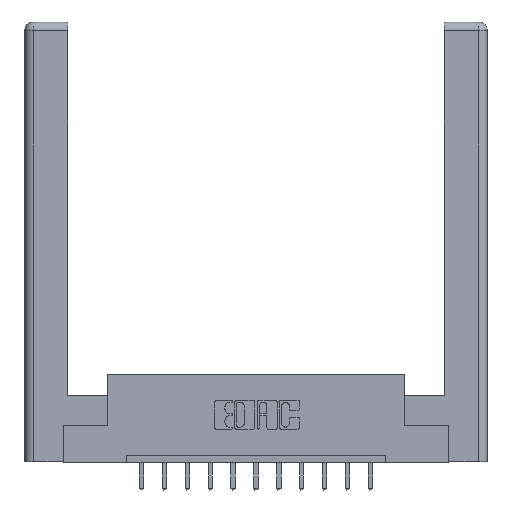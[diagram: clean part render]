
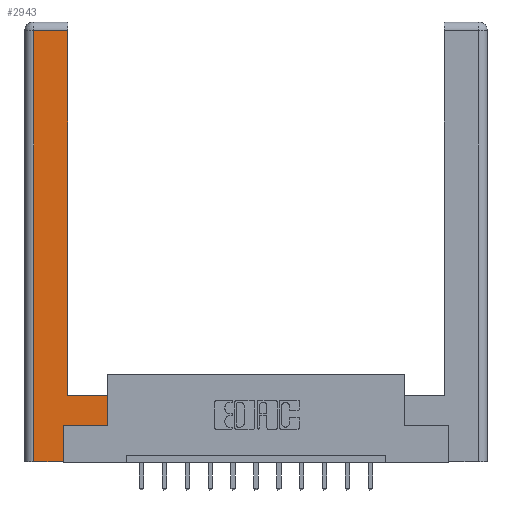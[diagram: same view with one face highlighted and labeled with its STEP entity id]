
A CAD part, top view. The second image highlights one B-rep face of the part: STEP entity #2943.
In plain terms, the highlighted planar face has unit normal (0, 0, 1).
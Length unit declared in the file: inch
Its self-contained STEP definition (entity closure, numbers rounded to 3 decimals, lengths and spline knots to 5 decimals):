
#169 = ORIENTED_EDGE ( 'NONE', *, *, #5644, .T. ) ;
#477 = LINE ( 'NONE', #10671, #6953 ) ;
#510 = CARTESIAN_POINT ( 'NONE',  ( 0.0615, 0., 0. ) ) ;
#787 = ORIENTED_EDGE ( 'NONE', *, *, #1074, .T. ) ;
#793 = DIRECTION ( 'NONE',  ( 0., 1., 0. ) ) ;
#1074 = EDGE_CURVE ( 'NONE', #13514, #2244, #11296, .T. ) ;
#1350 = EDGE_CURVE ( 'NONE', #8315, #7139, #10539, .T. ) ;
#1423 = CARTESIAN_POINT ( 'NONE',  ( 0.565, 0.245, 0. ) ) ;
#1701 = CARTESIAN_POINT ( 'NONE',  ( 0.265, 0.245, 0. ) ) ;
#2244 = VERTEX_POINT ( 'NONE', #6016 ) ;
#2795 = VERTEX_POINT ( 'NONE', #6215 ) ;
#2849 = ORIENTED_EDGE ( 'NONE', *, *, #7097, .T. ) ;
#2943 = ADVANCED_FACE ( 'NONE', ( #5965 ), #5645, .F. ) ;
#3038 = AXIS2_PLACEMENT_3D ( 'NONE', #4341, #6858, #13749 ) ;
#3250 = CARTESIAN_POINT ( 'NONE',  ( 0.265, 0., 0. ) ) ;
#3886 = EDGE_CURVE ( 'NONE', #2244, #4468, #7607, .T. ) ;
#3928 = DIRECTION ( 'NONE',  ( 0., 1., 0. ) ) ;
#4077 = DIRECTION ( 'NONE',  ( 0., -1., 0. ) ) ;
#4226 = LINE ( 'NONE', #6475, #12362 ) ;
#4303 = DIRECTION ( 'NONE',  ( 0., 1., 0. ) ) ;
#4341 = CARTESIAN_POINT ( 'NONE',  ( 0., 0., 0. ) ) ;
#4468 = VERTEX_POINT ( 'NONE', #5887 ) ;
#4658 = LINE ( 'NONE', #5801, #8648 ) ;
#4665 = VERTEX_POINT ( 'NONE', #6940 ) ;
#5644 = EDGE_CURVE ( 'NONE', #2795, #13514, #4658, .T. ) ;
#5645 = PLANE ( 'NONE',  #3038 ) ;
#5801 = CARTESIAN_POINT ( 'NONE',  ( 0.0615, 2.94, 0. ) ) ;
#5887 = CARTESIAN_POINT ( 'NONE',  ( 0.265, 0., 0. ) ) ;
#5965 = FACE_OUTER_BOUND ( 'NONE', #11839, .T. ) ;
#6016 = CARTESIAN_POINT ( 'NONE',  ( 0.0615, 0., 0. ) ) ;
#6047 = DIRECTION ( 'NONE',  ( 1., 0., 0. ) ) ;
#6215 = CARTESIAN_POINT ( 'NONE',  ( 0.295, 2.94, 0. ) ) ;
#6428 = CARTESIAN_POINT ( 'NONE',  ( 0.295, 3., 0. ) ) ;
#6475 = CARTESIAN_POINT ( 'NONE',  ( 0.565, 0.45, 0. ) ) ;
#6858 = DIRECTION ( 'NONE',  ( 0., 0., -1. ) ) ;
#6902 = ORIENTED_EDGE ( 'NONE', *, *, #7715, .T. ) ;
#6940 = CARTESIAN_POINT ( 'NONE',  ( 0.565, 0.45, 0. ) ) ;
#6953 = VECTOR ( 'NONE', #11708, 39.37008 ) ;
#7097 = EDGE_CURVE ( 'NONE', #4468, #8315, #10966, .T. ) ;
#7139 = VERTEX_POINT ( 'NONE', #11081 ) ;
#7479 = VECTOR ( 'NONE', #6047, 39.37008 ) ;
#7607 = LINE ( 'NONE', #3250, #9777 ) ;
#7690 = LINE ( 'NONE', #6428, #13665 ) ;
#7715 = EDGE_CURVE ( 'NONE', #9629, #2795, #7690, .T. ) ;
#7889 = VECTOR ( 'NONE', #3928, 39.37008 ) ;
#8315 = VERTEX_POINT ( 'NONE', #14630 ) ;
#8424 = ORIENTED_EDGE ( 'NONE', *, *, #1350, .T. ) ;
#8648 = VECTOR ( 'NONE', #11890, 39.37008 ) ;
#9366 = ORIENTED_EDGE ( 'NONE', *, *, #14940, .T. ) ;
#9485 = VECTOR ( 'NONE', #4077, 39.37008 ) ;
#9629 = VERTEX_POINT ( 'NONE', #13141 ) ;
#9777 = VECTOR ( 'NONE', #12495, 39.37008 ) ;
#10189 = ORIENTED_EDGE ( 'NONE', *, *, #3886, .T. ) ;
#10539 = LINE ( 'NONE', #1423, #7479 ) ;
#10671 = CARTESIAN_POINT ( 'NONE',  ( 0.295, 0.45, 0. ) ) ;
#10966 = LINE ( 'NONE', #1701, #7889 ) ;
#11081 = CARTESIAN_POINT ( 'NONE',  ( 0.565, 0.245, 0. ) ) ;
#11296 = LINE ( 'NONE', #510, #9485 ) ;
#11708 = DIRECTION ( 'NONE',  ( -1., 0., 0. ) ) ;
#11783 = ORIENTED_EDGE ( 'NONE', *, *, #14188, .T. ) ;
#11839 = EDGE_LOOP ( 'NONE', ( #6902, #169, #787, #10189, #2849, #8424, #9366, #11783 ) ) ;
#11890 = DIRECTION ( 'NONE',  ( -1., 0., 0. ) ) ;
#12362 = VECTOR ( 'NONE', #4303, 39.37008 ) ;
#12495 = DIRECTION ( 'NONE',  ( 1., 0., 0. ) ) ;
#13024 = CARTESIAN_POINT ( 'NONE',  ( 0.0615, 2.94, 0. ) ) ;
#13141 = CARTESIAN_POINT ( 'NONE',  ( 0.295, 0.45, 0. ) ) ;
#13514 = VERTEX_POINT ( 'NONE', #13024 ) ;
#13665 = VECTOR ( 'NONE', #793, 39.37008 ) ;
#13749 = DIRECTION ( 'NONE',  ( -1., 0., 0. ) ) ;
#14188 = EDGE_CURVE ( 'NONE', #4665, #9629, #477, .T. ) ;
#14630 = CARTESIAN_POINT ( 'NONE',  ( 0.265, 0.245, 0. ) ) ;
#14940 = EDGE_CURVE ( 'NONE', #7139, #4665, #4226, .T. ) ;
